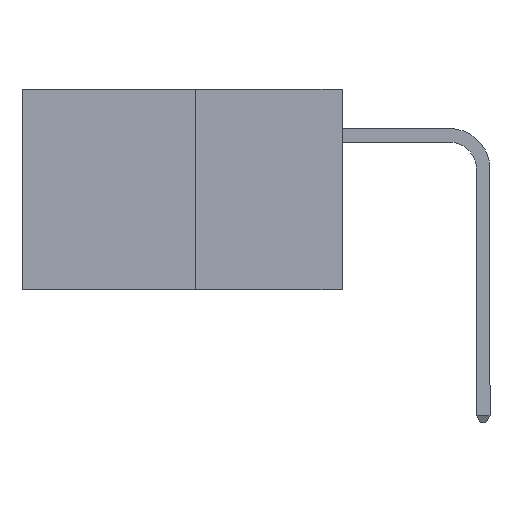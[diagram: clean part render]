
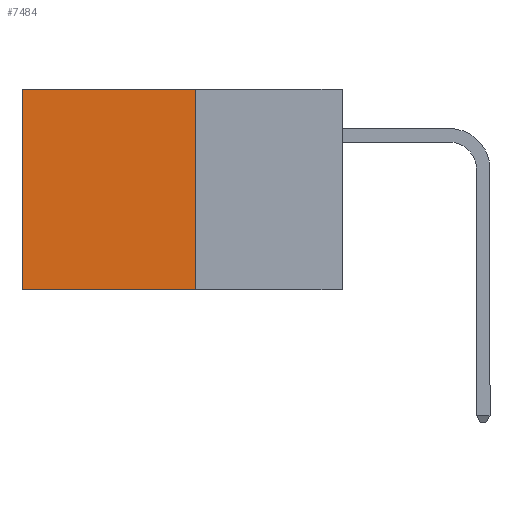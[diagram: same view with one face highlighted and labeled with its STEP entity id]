
A CAD part, left-side view. The second image highlights one B-rep face of the part: STEP entity #7484.
In plain terms, the highlighted planar face has unit normal (-1, 0, 0).
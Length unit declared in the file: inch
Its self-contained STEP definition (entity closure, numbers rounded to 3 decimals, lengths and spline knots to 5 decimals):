
#446 = VERTEX_POINT ( 'NONE', #730 ) ;
#730 = CARTESIAN_POINT ( 'NONE',  ( 0.277, 0.27, 0. ) ) ;
#909 = CARTESIAN_POINT ( 'NONE',  ( 0.277, 0.27, -0.37 ) ) ;
#924 = LINE ( 'NONE', #2664, #7998 ) ;
#932 = CARTESIAN_POINT ( 'NONE',  ( 0.277, 0.27, 0. ) ) ;
#941 = DIRECTION ( 'NONE',  ( 0., 1., 0. ) ) ;
#1064 = DIRECTION ( 'NONE',  ( 0., 0., -1. ) ) ;
#1329 = DIRECTION ( 'NONE',  ( 0., 0., -1. ) ) ;
#1347 = DIRECTION ( 'NONE',  ( 1., 0., 0. ) ) ;
#1434 = PLANE ( 'NONE',  #5876 ) ;
#1539 = CARTESIAN_POINT ( 'NONE',  ( 0.277, 0.27, -0.37 ) ) ;
#2628 = DIRECTION ( 'NONE',  ( 0., 1., 0. ) ) ;
#2664 = CARTESIAN_POINT ( 'NONE',  ( 0.277, 0.27, -0.37 ) ) ;
#3176 = ORIENTED_EDGE ( 'NONE', *, *, #7550, .T. ) ;
#3187 = ORIENTED_EDGE ( 'NONE', *, *, #4293, .F. ) ;
#3239 = FACE_OUTER_BOUND ( 'NONE', #5004, .T. ) ;
#3407 = VECTOR ( 'NONE', #1064, 39.37008 ) ;
#3923 = VERTEX_POINT ( 'NONE', #4175 ) ;
#4081 = ORIENTED_EDGE ( 'NONE', *, *, #6173, .F. ) ;
#4175 = CARTESIAN_POINT ( 'NONE',  ( 0.277, 0.27, -0.37 ) ) ;
#4239 = VECTOR ( 'NONE', #941, 39.37008 ) ;
#4293 = EDGE_CURVE ( 'NONE', #446, #3923, #7021, .T. ) ;
#4318 = CARTESIAN_POINT ( 'NONE',  ( 0.277, 0.59, 0. ) ) ;
#5004 = EDGE_LOOP ( 'NONE', ( #5195, #4081, #3187, #3176 ) ) ;
#5034 = EDGE_CURVE ( 'NONE', #5672, #6626, #6913, .T. ) ;
#5161 = VECTOR ( 'NONE', #7579, 39.37008 ) ;
#5195 = ORIENTED_EDGE ( 'NONE', *, *, #5034, .T. ) ;
#5672 = VERTEX_POINT ( 'NONE', #4318 ) ;
#5876 = AXIS2_PLACEMENT_3D ( 'NONE', #1539, #1347, #1329 ) ;
#6173 = EDGE_CURVE ( 'NONE', #3923, #6626, #924, .T. ) ;
#6626 = VERTEX_POINT ( 'NONE', #7350 ) ;
#6913 = LINE ( 'NONE', #7601, #5161 ) ;
#7021 = LINE ( 'NONE', #909, #3407 ) ;
#7350 = CARTESIAN_POINT ( 'NONE',  ( 0.277, 0.59, -0.37 ) ) ;
#7484 = ADVANCED_FACE ( 'NONE', ( #3239 ), #1434, .F. ) ;
#7550 = EDGE_CURVE ( 'NONE', #446, #5672, #7899, .T. ) ;
#7579 = DIRECTION ( 'NONE',  ( 0., 0., -1. ) ) ;
#7601 = CARTESIAN_POINT ( 'NONE',  ( 0.277, 0.59, -0.37 ) ) ;
#7899 = LINE ( 'NONE', #932, #4239 ) ;
#7998 = VECTOR ( 'NONE', #2628, 39.37008 ) ;
